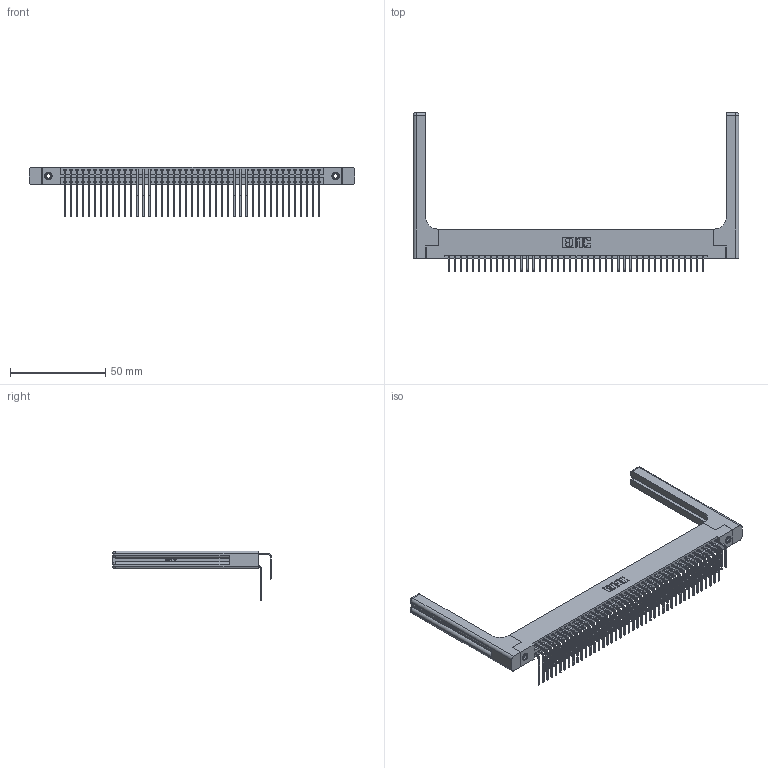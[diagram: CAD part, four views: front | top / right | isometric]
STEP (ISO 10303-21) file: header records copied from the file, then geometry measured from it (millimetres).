
FILE_DESCRIPTION (( 'STEP AP203' ), '1' );
FILE_NAME ('396-086-558-258.STEP', '2019-11-03T13:34:02', ( '' ), ( '' ), 'SwSTEP 2.0', 'SolidWorks 2016', '' );
FILE_SCHEMA (( 'CONFIG_CONTROL_DESIGN' ));
Length unit declared in the file: inch
Products named in the file (6): 346 Part_Flush Mounting Lugs - 0.156 Dia-TH; 346-220-058_345-220-058; 396-086-558-258; 345-292-001_558 559 Tail - 1; 345-250-001_345-250-001-102; 345-292-001_558 Tail - 2
Assembly tree (91 placements, depth 2):
  396-086-558-258
    346 Part_Flush Mounting Lugs - 0.156 Dia-TH
    345-292-001_558 559 Tail - 1  x43
    345-292-001_558 Tail - 2  x43
    345-250-001_345-250-001-102  x2
    346-220-058_345-220-058  x2
Bounding box: 170.59 x 83.12 x 26.16 mm (x, y, z)
Volume: 24632.4 mm3; surface area: 30926.1 mm2
Topology: 91 solids, 91 shells, 5022 faces, 14841 edges, 9758 vertices
Faces by surface type: plane 3406, cylinder 1556, bspline 36, cone 12, sphere 8, torus 4
Entity records: 34894 total; most frequent: CARTESIAN_POINT 6808, ORIENTED_EDGE 5488, DIRECTION 4956, EDGE_CURVE 2744, VECTOR 2308, LINE 2308, VERTEX_POINT 1818, AXIS2_PLACEMENT_3D 1324
